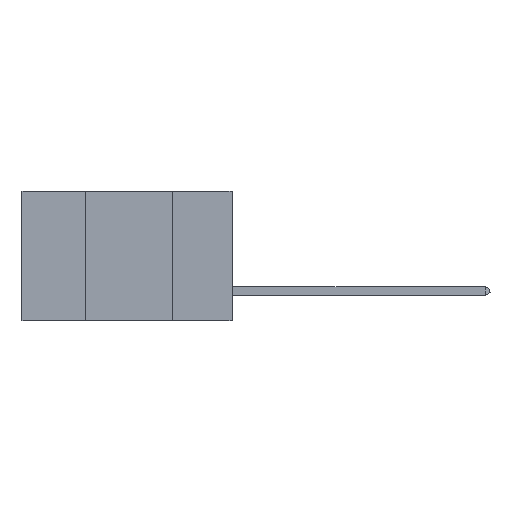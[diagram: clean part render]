
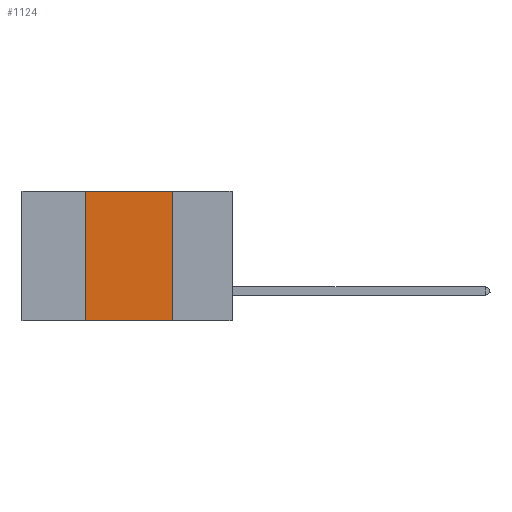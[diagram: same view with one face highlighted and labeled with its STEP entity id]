
A CAD part, left-side view. The second image highlights one B-rep face of the part: STEP entity #1124.
In plain terms, the highlighted planar face has unit normal (-1, 0, 0).
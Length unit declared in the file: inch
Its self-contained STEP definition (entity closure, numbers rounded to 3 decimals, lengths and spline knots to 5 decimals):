
#298 = EDGE_CURVE ( 'NONE', #13491, #3043, #15696, .T. ) ;
#493 = ORIENTED_EDGE ( 'NONE', *, *, #15456, .T. ) ;
#1124 = ADVANCED_FACE ( 'NONE', ( #7382 ), #11006, .F. ) ;
#1459 = LINE ( 'NONE', #17185, #10478 ) ;
#2644 = DIRECTION ( 'NONE',  ( 0., 0., -1. ) ) ;
#2746 = CARTESIAN_POINT ( 'NONE',  ( 0., 0.17, -0.37 ) ) ;
#2892 = VECTOR ( 'NONE', #13050, 39.37008 ) ;
#3043 = VERTEX_POINT ( 'NONE', #12292 ) ;
#3923 = VECTOR ( 'NONE', #2644, 39.37008 ) ;
#4258 = VERTEX_POINT ( 'NONE', #16060 ) ;
#5021 = LINE ( 'NONE', #15977, #17071 ) ;
#5158 = DIRECTION ( 'NONE',  ( 1., 0., 0. ) ) ;
#6461 = CARTESIAN_POINT ( 'NONE',  ( 0., 0.6, 0. ) ) ;
#6639 = AXIS2_PLACEMENT_3D ( 'NONE', #6461, #5158, #8091 ) ;
#6982 = EDGE_CURVE ( 'NONE', #4258, #11315, #9985, .T. ) ;
#7230 = ORIENTED_EDGE ( 'NONE', *, *, #298, .F. ) ;
#7293 = CARTESIAN_POINT ( 'NONE',  ( 0., 0.42, -0.37 ) ) ;
#7382 = FACE_OUTER_BOUND ( 'NONE', #15487, .T. ) ;
#7393 = DIRECTION ( 'NONE',  ( 0., -1., 0. ) ) ;
#7750 = CARTESIAN_POINT ( 'NONE',  ( 0., 0.17, 0. ) ) ;
#8091 = DIRECTION ( 'NONE',  ( 0., 0., -1. ) ) ;
#9985 = LINE ( 'NONE', #7750, #3923 ) ;
#10478 = VECTOR ( 'NONE', #17245, 39.37008 ) ;
#10945 = ORIENTED_EDGE ( 'NONE', *, *, #12235, .F. ) ;
#11006 = PLANE ( 'NONE',  #6639 ) ;
#11315 = VERTEX_POINT ( 'NONE', #2746 ) ;
#12235 = EDGE_CURVE ( 'NONE', #3043, #4258, #5021, .T. ) ;
#12292 = CARTESIAN_POINT ( 'NONE',  ( 0., 0.42, 0. ) ) ;
#13050 = DIRECTION ( 'NONE',  ( 0., 0., 1. ) ) ;
#13304 = CARTESIAN_POINT ( 'NONE',  ( 0., 0.42, 0. ) ) ;
#13491 = VERTEX_POINT ( 'NONE', #7293 ) ;
#15456 = EDGE_CURVE ( 'NONE', #13491, #11315, #1459, .T. ) ;
#15487 = EDGE_LOOP ( 'NONE', ( #17810, #10945, #7230, #493 ) ) ;
#15696 = LINE ( 'NONE', #13304, #2892 ) ;
#15977 = CARTESIAN_POINT ( 'NONE',  ( 0., 0.6, 0. ) ) ;
#16060 = CARTESIAN_POINT ( 'NONE',  ( 0., 0.17, 0. ) ) ;
#17071 = VECTOR ( 'NONE', #7393, 39.37008 ) ;
#17185 = CARTESIAN_POINT ( 'NONE',  ( 0., 0.6, -0.37 ) ) ;
#17245 = DIRECTION ( 'NONE',  ( 0., -1., 0. ) ) ;
#17810 = ORIENTED_EDGE ( 'NONE', *, *, #6982, .F. ) ;
